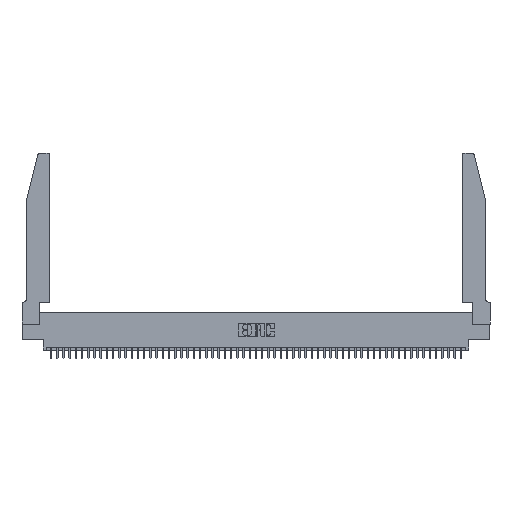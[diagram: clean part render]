
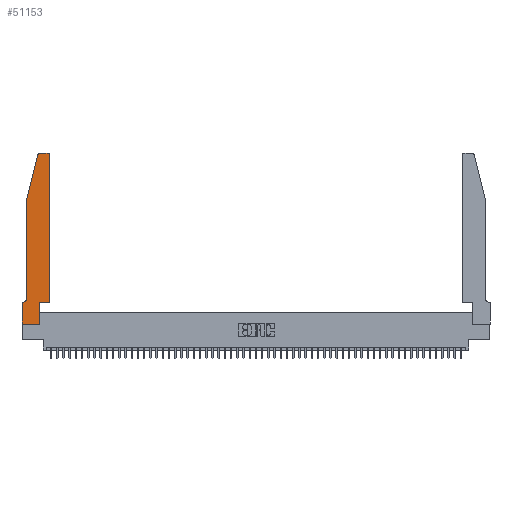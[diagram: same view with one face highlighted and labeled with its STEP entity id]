
A CAD part, top view. The second image highlights one B-rep face of the part: STEP entity #51153.
In plain terms, the highlighted planar face has unit normal (0, 0, 1).
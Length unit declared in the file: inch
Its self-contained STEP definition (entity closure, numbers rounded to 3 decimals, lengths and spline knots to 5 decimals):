
#2331 = EDGE_CURVE ( 'NONE', #2682, #28260, #31679, .T. ) ;
#2391 = DIRECTION ( 'NONE',  ( 1., 0., 0. ) ) ;
#2452 = VECTOR ( 'NONE', #24865, 39.37008 ) ;
#2523 = DIRECTION ( 'NONE',  ( 0., 0., 1. ) ) ;
#2565 = VECTOR ( 'NONE', #15168, 39.37008 ) ;
#2682 = VERTEX_POINT ( 'NONE', #42690 ) ;
#3215 = VERTEX_POINT ( 'NONE', #5553 ) ;
#4651 = LINE ( 'NONE', #33103, #8568 ) ;
#5553 = CARTESIAN_POINT ( 'NONE',  ( 0.0755, 0.42, 0.37 ) ) ;
#5631 = LINE ( 'NONE', #50293, #23229 ) ;
#6531 = AXIS2_PLACEMENT_3D ( 'NONE', #44483, #2523, #19646 ) ;
#6621 = EDGE_CURVE ( 'NONE', #28260, #10117, #21913, .T. ) ;
#6647 = CARTESIAN_POINT ( 'NONE',  ( 0., 0., 0.37 ) ) ;
#6906 = DIRECTION ( 'NONE',  ( 0., 0., -1. ) ) ;
#7073 = CARTESIAN_POINT ( 'NONE',  ( 0.4205, 2.75, 0.37 ) ) ;
#7413 = EDGE_LOOP ( 'NONE', ( #34867, #43333, #19874, #13007, #8040, #10178, #25681, #21731, #45899, #12020, #17842, #13152 ) ) ;
#7927 = FACE_OUTER_BOUND ( 'NONE', #7413, .T. ) ;
#8040 = ORIENTED_EDGE ( 'NONE', *, *, #47926, .T. ) ;
#8128 = LINE ( 'NONE', #34719, #44077 ) ;
#8496 = CARTESIAN_POINT ( 'NONE',  ( 0.2865, 0.35, 0.37 ) ) ;
#8568 = VECTOR ( 'NONE', #45732, 39.37008 ) ;
#8855 = CARTESIAN_POINT ( 'NONE',  ( 0.4505, 0.35, 0.37 ) ) ;
#9180 = DIRECTION ( 'NONE',  ( -0.239, -0.971, 0. ) ) ;
#9373 = CARTESIAN_POINT ( 'NONE',  ( 0.0755, 2., 0.37 ) ) ;
#10054 = AXIS2_PLACEMENT_3D ( 'NONE', #10590, #19677, #2391 ) ;
#10117 = VERTEX_POINT ( 'NONE', #13276 ) ;
#10178 = ORIENTED_EDGE ( 'NONE', *, *, #2331, .T. ) ;
#10590 = CARTESIAN_POINT ( 'NONE',  ( 0.4205, 2.72, 0.37 ) ) ;
#11497 = CARTESIAN_POINT ( 'NONE',  ( 0.25487, 2.72718, 0.37 ) ) ;
#12020 = ORIENTED_EDGE ( 'NONE', *, *, #37830, .T. ) ;
#13007 = ORIENTED_EDGE ( 'NONE', *, *, #14006, .T. ) ;
#13152 = ORIENTED_EDGE ( 'NONE', *, *, #27652, .T. ) ;
#13276 = CARTESIAN_POINT ( 'NONE',  ( 0., 0., 0.37 ) ) ;
#13466 = VECTOR ( 'NONE', #27931, 39.37008 ) ;
#14006 = EDGE_CURVE ( 'NONE', #26744, #3215, #4651, .T. ) ;
#14774 = VERTEX_POINT ( 'NONE', #42555 ) ;
#15168 = DIRECTION ( 'NONE',  ( 1., 0., 0. ) ) ;
#15334 = DIRECTION ( 'NONE',  ( 1., 0., 0. ) ) ;
#15393 = CARTESIAN_POINT ( 'NONE',  ( 0.284, 2.75, 0.37 ) ) ;
#15530 = LINE ( 'NONE', #49815, #2452 ) ;
#15943 = VECTOR ( 'NONE', #41912, 39.37008 ) ;
#16673 = VECTOR ( 'NONE', #50616, 39.37008 ) ;
#17146 = CARTESIAN_POINT ( 'NONE',  ( 0.0755, 0.35, 0.37 ) ) ;
#17842 = ORIENTED_EDGE ( 'NONE', *, *, #28429, .T. ) ;
#19646 = DIRECTION ( 'NONE',  ( 1., 0., 0. ) ) ;
#19677 = DIRECTION ( 'NONE',  ( 0., 0., 1. ) ) ;
#19874 = ORIENTED_EDGE ( 'NONE', *, *, #28435, .T. ) ;
#20329 = VERTEX_POINT ( 'NONE', #11497 ) ;
#20985 = DIRECTION ( 'NONE',  ( -1., 0., 0. ) ) ;
#21305 = VERTEX_POINT ( 'NONE', #22494 ) ;
#21731 = ORIENTED_EDGE ( 'NONE', *, *, #42588, .T. ) ;
#21913 = LINE ( 'NONE', #6647, #13466 ) ;
#21923 = DIRECTION ( 'NONE',  ( 0., 1., 0. ) ) ;
#22133 = CARTESIAN_POINT ( 'NONE',  ( 0.2865, 0., 0.37 ) ) ;
#22158 = AXIS2_PLACEMENT_3D ( 'NONE', #27503, #36293, #15334 ) ;
#22494 = CARTESIAN_POINT ( 'NONE',  ( 0.2865, 0.35, 0.37 ) ) ;
#23229 = VECTOR ( 'NONE', #20985, 39.37008 ) ;
#24865 = DIRECTION ( 'NONE',  ( 1., 0., 0. ) ) ;
#25678 = LINE ( 'NONE', #8496, #15943 ) ;
#25681 = ORIENTED_EDGE ( 'NONE', *, *, #6621, .T. ) ;
#26744 = VERTEX_POINT ( 'NONE', #39503 ) ;
#27503 = CARTESIAN_POINT ( 'NONE',  ( 0.284, 2.72, 0.37 ) ) ;
#27652 = EDGE_CURVE ( 'NONE', #14774, #41426, #46129, .T. ) ;
#27666 = VECTOR ( 'NONE', #9180, 39.37008 ) ;
#27931 = DIRECTION ( 'NONE',  ( 0., -1., 0. ) ) ;
#28260 = VERTEX_POINT ( 'NONE', #53425 ) ;
#28429 = EDGE_CURVE ( 'NONE', #37966, #14774, #8128, .T. ) ;
#28435 = EDGE_CURVE ( 'NONE', #20329, #26744, #45377, .T. ) ;
#29640 = EDGE_CURVE ( 'NONE', #44063, #21305, #25678, .T. ) ;
#31679 = LINE ( 'NONE', #17146, #16673 ) ;
#33103 = CARTESIAN_POINT ( 'NONE',  ( 0.0755, 2., 0.37 ) ) ;
#34719 = CARTESIAN_POINT ( 'NONE',  ( 0.4505, 0.35, 0.37 ) ) ;
#34867 = ORIENTED_EDGE ( 'NONE', *, *, #38476, .T. ) ;
#35915 = DIRECTION ( 'NONE',  ( -1., 0., 0. ) ) ;
#35956 = CARTESIAN_POINT ( 'NONE',  ( 0., 0., 0.37 ) ) ;
#36293 = DIRECTION ( 'NONE',  ( 0., 0., 1. ) ) ;
#37105 = EDGE_CURVE ( 'NONE', #49972, #20329, #51036, .T. ) ;
#37830 = EDGE_CURVE ( 'NONE', #21305, #37966, #15530, .T. ) ;
#37966 = VERTEX_POINT ( 'NONE', #8855 ) ;
#38476 = EDGE_CURVE ( 'NONE', #41426, #49972, #5631, .T. ) ;
#39503 = CARTESIAN_POINT ( 'NONE',  ( 0.0755, 2., 0.37 ) ) ;
#40414 = LINE ( 'NONE', #35956, #2565 ) ;
#41426 = VERTEX_POINT ( 'NONE', #7073 ) ;
#41912 = DIRECTION ( 'NONE',  ( 0., 1., 0. ) ) ;
#42555 = CARTESIAN_POINT ( 'NONE',  ( 0.4505, 2.72, 0.37 ) ) ;
#42588 = EDGE_CURVE ( 'NONE', #10117, #44063, #40414, .T. ) ;
#42690 = CARTESIAN_POINT ( 'NONE',  ( 0.0055, 0.35, 0.37 ) ) ;
#43183 = AXIS2_PLACEMENT_3D ( 'NONE', #44513, #6906, #35915 ) ;
#43333 = ORIENTED_EDGE ( 'NONE', *, *, #37105, .T. ) ;
#44063 = VERTEX_POINT ( 'NONE', #22133 ) ;
#44077 = VECTOR ( 'NONE', #21923, 39.37008 ) ;
#44483 = CARTESIAN_POINT ( 'NONE',  ( 0., 0.35, 0.37 ) ) ;
#44513 = CARTESIAN_POINT ( 'NONE',  ( 0.0055, 0.42, 0.37 ) ) ;
#44675 = PLANE ( 'NONE',  #6531 ) ;
#45377 = LINE ( 'NONE', #9373, #27666 ) ;
#45732 = DIRECTION ( 'NONE',  ( 0., -1., 0. ) ) ;
#45899 = ORIENTED_EDGE ( 'NONE', *, *, #29640, .T. ) ;
#46129 = CIRCLE ( 'NONE', #10054, 0.03 ) ;
#47926 = EDGE_CURVE ( 'NONE', #3215, #2682, #52637, .T. ) ;
#49815 = CARTESIAN_POINT ( 'NONE',  ( 0.4505, 0.35, 0.37 ) ) ;
#49972 = VERTEX_POINT ( 'NONE', #15393 ) ;
#50293 = CARTESIAN_POINT ( 'NONE',  ( 0.2605, 2.75, 0.37 ) ) ;
#50616 = DIRECTION ( 'NONE',  ( -1., 0., 0. ) ) ;
#51036 = CIRCLE ( 'NONE', #22158, 0.03 ) ;
#51153 = ADVANCED_FACE ( 'NONE', ( #7927 ), #44675, .T. ) ;
#52637 = CIRCLE ( 'NONE', #43183, 0.07 ) ;
#53425 = CARTESIAN_POINT ( 'NONE',  ( 0., 0.35, 0.37 ) ) ;
